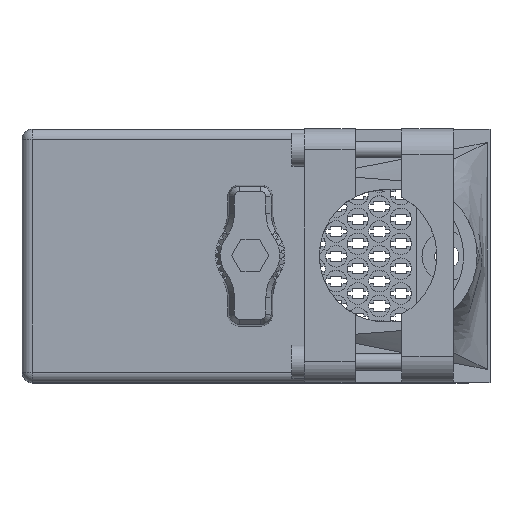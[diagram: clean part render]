
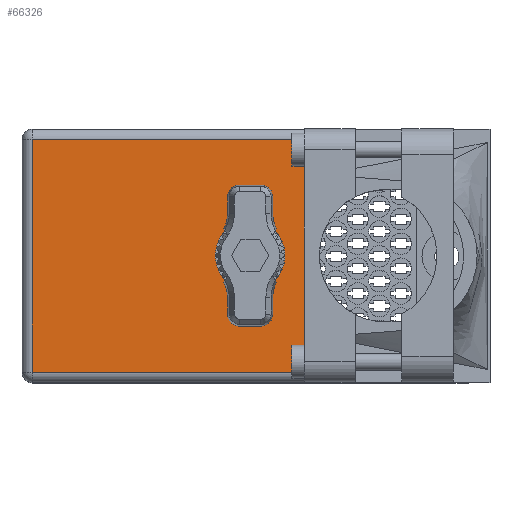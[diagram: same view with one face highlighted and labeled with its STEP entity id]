
A CAD part, top view. The second image highlights one B-rep face of the part: STEP entity #66326.
In plain terms, the highlighted face is planar.
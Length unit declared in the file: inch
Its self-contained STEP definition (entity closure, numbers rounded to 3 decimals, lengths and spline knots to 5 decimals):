
#86 = DIRECTION ( 'NONE',  ( 0., 0., 1. ) ) ;
#4081 = DIRECTION ( 'NONE',  ( 0., 0., 1. ) ) ;
#5415 = CARTESIAN_POINT ( 'NONE',  ( 0.3275, 1.93, 0.703 ) ) ;
#9628 = CARTESIAN_POINT ( 'NONE',  ( 0., 1.93, 0.17 ) ) ;
#18530 = FACE_OUTER_BOUND ( 'NONE', #21289, .T. ) ;
#18703 = VERTEX_POINT ( 'NONE', #70694 ) ;
#21289 = EDGE_LOOP ( 'NONE', ( #48203, #92497, #51426, #93309 ) ) ;
#22151 = ORIENTED_EDGE ( 'NONE', *, *, #30168, .F. ) ;
#26016 = EDGE_CURVE ( 'NONE', #62588, #27218, #35431, .T. ) ;
#27218 = VERTEX_POINT ( 'NONE', #61264 ) ;
#28711 = EDGE_CURVE ( 'NONE', #87668, #27218, #85317, .T. ) ;
#28781 = DIRECTION ( 'NONE',  ( -1., 0., 0. ) ) ;
#29726 = CARTESIAN_POINT ( 'NONE',  ( -1.3155, 1.93, -0.703 ) ) ;
#30168 = EDGE_CURVE ( 'NONE', #18703, #40978, #41831, .T. ) ;
#34070 = LINE ( 'NONE', #90347, #93873 ) ;
#35426 = DIRECTION ( 'NONE',  ( 0., 1., 0. ) ) ;
#35431 = LINE ( 'NONE', #5415, #89314 ) ;
#37306 = DIRECTION ( 'NONE',  ( 1., 0., 0. ) ) ;
#40491 = VECTOR ( 'NONE', #86, 39.37008 ) ;
#40978 = VERTEX_POINT ( 'NONE', #9628 ) ;
#41831 = CIRCLE ( 'NONE', #82117, 0.17 ) ;
#42493 = DIRECTION ( 'NONE',  ( 0., 0., 1. ) ) ;
#43215 = CARTESIAN_POINT ( 'NONE',  ( 0., 1.93, 0. ) ) ;
#48203 = ORIENTED_EDGE ( 'NONE', *, *, #65640, .T. ) ;
#50731 = CARTESIAN_POINT ( 'NONE',  ( 0.3275, 1.93, -0.765 ) ) ;
#51426 = ORIENTED_EDGE ( 'NONE', *, *, #28711, .F. ) ;
#54546 = FACE_BOUND ( 'NONE', #93365, .T. ) ;
#57308 = DIRECTION ( 'NONE',  ( 0., 1., 0. ) ) ;
#57960 = CARTESIAN_POINT ( 'NONE',  ( 0., 1.93, 0. ) ) ;
#58009 = DIRECTION ( 'NONE',  ( 0., 0., 1. ) ) ;
#59467 = ORIENTED_EDGE ( 'NONE', *, *, #63832, .F. ) ;
#60873 = LINE ( 'NONE', #84259, #40491 ) ;
#61264 = CARTESIAN_POINT ( 'NONE',  ( 0.3275, 1.93, 0.703 ) ) ;
#62588 = VERTEX_POINT ( 'NONE', #97019 ) ;
#63832 = EDGE_CURVE ( 'NONE', #40978, #18703, #76563, .T. ) ;
#64500 = VERTEX_POINT ( 'NONE', #29726 ) ;
#65640 = EDGE_CURVE ( 'NONE', #64500, #62588, #60873, .T. ) ;
#66326 = ADVANCED_FACE ( 'NONE', ( #18530, #54546 ), #81346, .T. ) ;
#70694 = CARTESIAN_POINT ( 'NONE',  ( 0., 1.93, -0.17 ) ) ;
#74651 = CARTESIAN_POINT ( 'NONE',  ( -1.3775, 1.93, -0.765 ) ) ;
#76563 = CIRCLE ( 'NONE', #85274, 0.17 ) ;
#81346 = PLANE ( 'NONE',  #81653 ) ;
#81653 = AXIS2_PLACEMENT_3D ( 'NONE', #74651, #35426, #81987 ) ;
#81987 = DIRECTION ( 'NONE',  ( -1., 0., 0. ) ) ;
#82117 = AXIS2_PLACEMENT_3D ( 'NONE', #57960, #57308, #42493 ) ;
#84259 = CARTESIAN_POINT ( 'NONE',  ( -1.3155, 1.93, -0.765 ) ) ;
#85274 = AXIS2_PLACEMENT_3D ( 'NONE', #43215, #96712, #58009 ) ;
#85317 = LINE ( 'NONE', #50731, #98386 ) ;
#87668 = VERTEX_POINT ( 'NONE', #94961 ) ;
#89314 = VECTOR ( 'NONE', #37306, 39.37008 ) ;
#90347 = CARTESIAN_POINT ( 'NONE',  ( -1.3775, 1.93, -0.703 ) ) ;
#92497 = ORIENTED_EDGE ( 'NONE', *, *, #26016, .T. ) ;
#93309 = ORIENTED_EDGE ( 'NONE', *, *, #94218, .T. ) ;
#93365 = EDGE_LOOP ( 'NONE', ( #59467, #22151 ) ) ;
#93873 = VECTOR ( 'NONE', #28781, 39.37008 ) ;
#94218 = EDGE_CURVE ( 'NONE', #87668, #64500, #34070, .T. ) ;
#94961 = CARTESIAN_POINT ( 'NONE',  ( 0.3275, 1.93, -0.703 ) ) ;
#96712 = DIRECTION ( 'NONE',  ( 0., 1., 0. ) ) ;
#97019 = CARTESIAN_POINT ( 'NONE',  ( -1.3155, 1.93, 0.703 ) ) ;
#98386 = VECTOR ( 'NONE', #4081, 39.37008 ) ;
